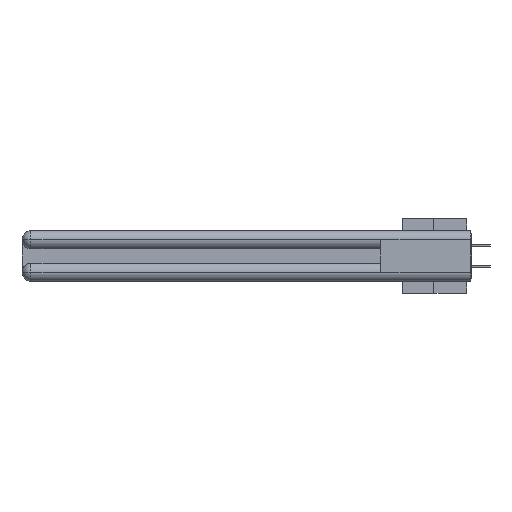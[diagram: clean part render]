
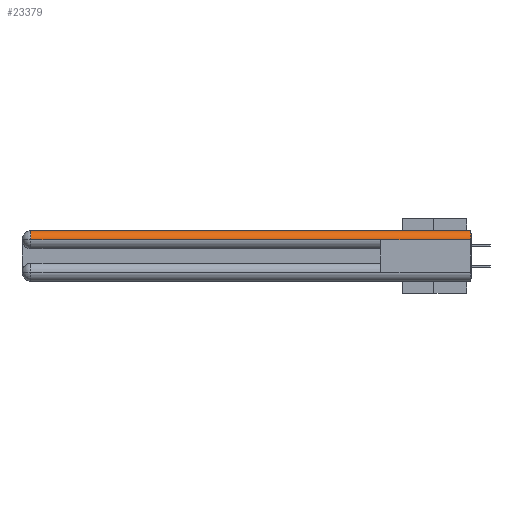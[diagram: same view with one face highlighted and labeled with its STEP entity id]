
A CAD part, left-side view. The second image highlights one B-rep face of the part: STEP entity #23379.
In plain terms, the highlighted cylindrical face has radius 1.562 mm (diameter 3.124 mm), a partial arc.
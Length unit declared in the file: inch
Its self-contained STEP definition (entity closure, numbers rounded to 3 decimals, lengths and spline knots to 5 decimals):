
#440 = VERTEX_POINT ( 'NONE', #1977 ) ;
#822 = CARTESIAN_POINT ( 'NONE',  ( 0.0615, 2.94, 0. ) ) ;
#1463 = CARTESIAN_POINT ( 'NONE',  ( 0.0615, 0., 0. ) ) ;
#1977 = CARTESIAN_POINT ( 'NONE',  ( 0.0615, 0., 0. ) ) ;
#3240 = CARTESIAN_POINT ( 'NONE',  ( 0., 2.94, -0.0615 ) ) ;
#5104 = CARTESIAN_POINT ( 'NONE',  ( 0.0615, 0., -0.0615 ) ) ;
#6972 = EDGE_CURVE ( 'NONE', #25073, #35726, #36732, .T. ) ;
#7395 = ORIENTED_EDGE ( 'NONE', *, *, #26906, .F. ) ;
#9079 = DIRECTION ( 'NONE',  ( 1., 0., 0. ) ) ;
#10818 = CARTESIAN_POINT ( 'NONE',  ( 0., 3., -0.0615 ) ) ;
#11007 = LINE ( 'NONE', #10818, #25798 ) ;
#11212 = AXIS2_PLACEMENT_3D ( 'NONE', #36196, #36717, #15426 ) ;
#11534 = ORIENTED_EDGE ( 'NONE', *, *, #27518, .F. ) ;
#12101 = CARTESIAN_POINT ( 'NONE',  ( 0., 0., -0.0615 ) ) ;
#13718 = DIRECTION ( 'NONE',  ( 0., -1., 0. ) ) ;
#15308 = EDGE_CURVE ( 'NONE', #35726, #22527, #11007, .T. ) ;
#15426 = DIRECTION ( 'NONE',  ( 0., 0., 1. ) ) ;
#17569 = DIRECTION ( 'NONE',  ( 0., 0., 1. ) ) ;
#18708 = CIRCLE ( 'NONE', #34524, 0.0615 ) ;
#18949 = CARTESIAN_POINT ( 'NONE',  ( 0., 0.6, -0.0615 ) ) ;
#19166 = CYLINDRICAL_SURFACE ( 'NONE', #20659, 0.0615 ) ;
#20108 = FACE_OUTER_BOUND ( 'NONE', #24355, .T. ) ;
#20659 = AXIS2_PLACEMENT_3D ( 'NONE', #5104, #22663, #17569 ) ;
#21704 = DIRECTION ( 'NONE',  ( 0., 1., 0. ) ) ;
#21957 = CARTESIAN_POINT ( 'NONE',  ( 0., 3., -0.0615 ) ) ;
#22456 = ORIENTED_EDGE ( 'NONE', *, *, #6972, .T. ) ;
#22527 = VERTEX_POINT ( 'NONE', #18949 ) ;
#22663 = DIRECTION ( 'NONE',  ( 0., 1., 0. ) ) ;
#23379 = ADVANCED_FACE ( 'NONE', ( #20108 ), #19166, .T. ) ;
#23489 = VECTOR ( 'NONE', #21704, 39.37008 ) ;
#24355 = EDGE_LOOP ( 'NONE', ( #24519, #22456, #37011, #7395, #11534 ) ) ;
#24519 = ORIENTED_EDGE ( 'NONE', *, *, #29358, .F. ) ;
#25073 = VERTEX_POINT ( 'NONE', #822 ) ;
#25798 = VECTOR ( 'NONE', #13718, 39.37008 ) ;
#26866 = VECTOR ( 'NONE', #28402, 39.37008 ) ;
#26906 = EDGE_CURVE ( 'NONE', #32256, #22527, #31585, .T. ) ;
#27518 = EDGE_CURVE ( 'NONE', #440, #32256, #18708, .T. ) ;
#28402 = DIRECTION ( 'NONE',  ( 0., -1., 0. ) ) ;
#29358 = EDGE_CURVE ( 'NONE', #25073, #440, #35925, .T. ) ;
#31585 = LINE ( 'NONE', #21957, #23489 ) ;
#32256 = VERTEX_POINT ( 'NONE', #12101 ) ;
#34524 = AXIS2_PLACEMENT_3D ( 'NONE', #39016, #39290, #9079 ) ;
#35726 = VERTEX_POINT ( 'NONE', #3240 ) ;
#35925 = LINE ( 'NONE', #1463, #26866 ) ;
#36196 = CARTESIAN_POINT ( 'NONE',  ( 0.0615, 2.94, -0.0615 ) ) ;
#36717 = DIRECTION ( 'NONE',  ( 0., -1., 0. ) ) ;
#36732 = CIRCLE ( 'NONE', #11212, 0.0615 ) ;
#37011 = ORIENTED_EDGE ( 'NONE', *, *, #15308, .T. ) ;
#39016 = CARTESIAN_POINT ( 'NONE',  ( 0.0615, 0., -0.0615 ) ) ;
#39290 = DIRECTION ( 'NONE',  ( 0., -1., 0. ) ) ;
